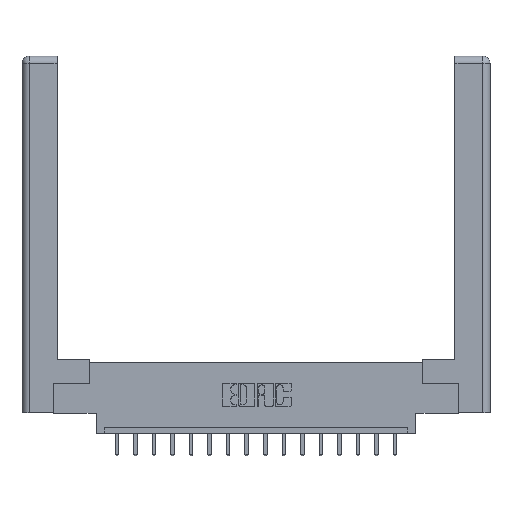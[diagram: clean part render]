
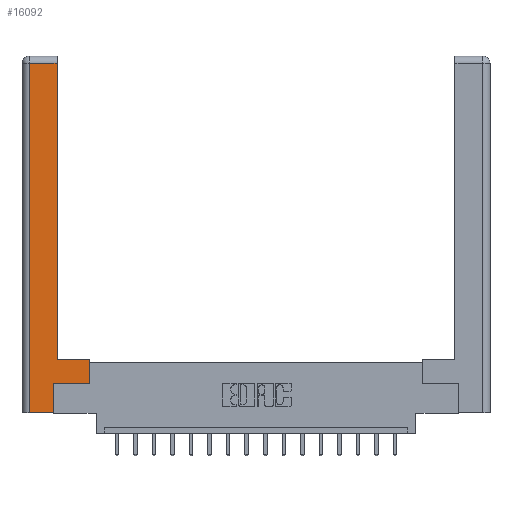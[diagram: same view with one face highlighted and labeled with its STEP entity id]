
A CAD part, top view. The second image highlights one B-rep face of the part: STEP entity #16092.
In plain terms, the highlighted planar face has unit normal (0, 0, 1).
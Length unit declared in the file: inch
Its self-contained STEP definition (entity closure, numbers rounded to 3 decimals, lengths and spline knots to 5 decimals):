
#26 = VECTOR ( 'NONE', #1888, 39.37008 ) ;
#117 = VERTEX_POINT ( 'NONE', #9153 ) ;
#232 = AXIS2_PLACEMENT_3D ( 'NONE', #5688, #18079, #15483 ) ;
#305 = CARTESIAN_POINT ( 'NONE',  ( 0.265, 0.245, 0. ) ) ;
#758 = DIRECTION ( 'NONE',  ( -1., 0., 0. ) ) ;
#790 = ORIENTED_EDGE ( 'NONE', *, *, #12209, .T. ) ;
#1109 = DIRECTION ( 'NONE',  ( -1., 0., 0. ) ) ;
#1177 = CARTESIAN_POINT ( 'NONE',  ( 0.295, 0.45, 0. ) ) ;
#1500 = CARTESIAN_POINT ( 'NONE',  ( 0.565, 0.245, 0. ) ) ;
#1694 = VECTOR ( 'NONE', #3540, 39.37008 ) ;
#1888 = DIRECTION ( 'NONE',  ( 1., 0., 0. ) ) ;
#2169 = LINE ( 'NONE', #305, #2615 ) ;
#2547 = VERTEX_POINT ( 'NONE', #9567 ) ;
#2615 = VECTOR ( 'NONE', #14109, 39.37008 ) ;
#2792 = ORIENTED_EDGE ( 'NONE', *, *, #10986, .T. ) ;
#3011 = CARTESIAN_POINT ( 'NONE',  ( 0.0615, 2.94, 0. ) ) ;
#3387 = CARTESIAN_POINT ( 'NONE',  ( 0.295, 3., 0. ) ) ;
#3540 = DIRECTION ( 'NONE',  ( 0., -1., 0. ) ) ;
#3660 = CARTESIAN_POINT ( 'NONE',  ( 0.0615, 0., 0. ) ) ;
#3812 = DIRECTION ( 'NONE',  ( 0., 1., 0. ) ) ;
#4677 = VECTOR ( 'NONE', #1109, 39.37008 ) ;
#4827 = VECTOR ( 'NONE', #12919, 39.37008 ) ;
#4859 = CARTESIAN_POINT ( 'NONE',  ( 0.295, 2.94, 0. ) ) ;
#4862 = VECTOR ( 'NONE', #758, 39.37008 ) ;
#5351 = CARTESIAN_POINT ( 'NONE',  ( 0.565, 0.245, 0. ) ) ;
#5362 = LINE ( 'NONE', #3387, #5566 ) ;
#5566 = VECTOR ( 'NONE', #7525, 39.37008 ) ;
#5688 = CARTESIAN_POINT ( 'NONE',  ( 0., 0., 0. ) ) ;
#6109 = VERTEX_POINT ( 'NONE', #17851 ) ;
#7306 = LINE ( 'NONE', #13396, #4862 ) ;
#7525 = DIRECTION ( 'NONE',  ( 0., 1., 0. ) ) ;
#7606 = FACE_OUTER_BOUND ( 'NONE', #17423, .T. ) ;
#7648 = ORIENTED_EDGE ( 'NONE', *, *, #13718, .T. ) ;
#8230 = CARTESIAN_POINT ( 'NONE',  ( 0.295, 0.45, 0. ) ) ;
#8294 = EDGE_CURVE ( 'NONE', #6109, #16015, #8418, .T. ) ;
#8418 = LINE ( 'NONE', #1177, #4677 ) ;
#8572 = LINE ( 'NONE', #1500, #4827 ) ;
#8828 = VERTEX_POINT ( 'NONE', #4859 ) ;
#8994 = EDGE_CURVE ( 'NONE', #9132, #6109, #12313, .T. ) ;
#9132 = VERTEX_POINT ( 'NONE', #5351 ) ;
#9153 = CARTESIAN_POINT ( 'NONE',  ( 0.0615, 0., 0. ) ) ;
#9270 = VECTOR ( 'NONE', #3812, 39.37008 ) ;
#9567 = CARTESIAN_POINT ( 'NONE',  ( 0.265, 0., 0. ) ) ;
#9794 = EDGE_CURVE ( 'NONE', #13438, #9132, #8572, .T. ) ;
#10761 = CARTESIAN_POINT ( 'NONE',  ( 0.265, 0.245, 0. ) ) ;
#10986 = EDGE_CURVE ( 'NONE', #16015, #8828, #5362, .T. ) ;
#11499 = VERTEX_POINT ( 'NONE', #3011 ) ;
#11604 = EDGE_CURVE ( 'NONE', #117, #2547, #12328, .T. ) ;
#12047 = ORIENTED_EDGE ( 'NONE', *, *, #14953, .T. ) ;
#12209 = EDGE_CURVE ( 'NONE', #8828, #11499, #7306, .T. ) ;
#12214 = LINE ( 'NONE', #3660, #1694 ) ;
#12313 = LINE ( 'NONE', #16367, #9270 ) ;
#12328 = LINE ( 'NONE', #14703, #26 ) ;
#12919 = DIRECTION ( 'NONE',  ( 1., 0., 0. ) ) ;
#13396 = CARTESIAN_POINT ( 'NONE',  ( 0.0615, 2.94, 0. ) ) ;
#13438 = VERTEX_POINT ( 'NONE', #10761 ) ;
#13718 = EDGE_CURVE ( 'NONE', #2547, #13438, #2169, .T. ) ;
#13885 = PLANE ( 'NONE',  #232 ) ;
#14109 = DIRECTION ( 'NONE',  ( 0., 1., 0. ) ) ;
#14703 = CARTESIAN_POINT ( 'NONE',  ( 0.265, 0., 0. ) ) ;
#14953 = EDGE_CURVE ( 'NONE', #11499, #117, #12214, .T. ) ;
#15483 = DIRECTION ( 'NONE',  ( -1., 0., 0. ) ) ;
#15624 = ORIENTED_EDGE ( 'NONE', *, *, #8294, .T. ) ;
#15806 = ORIENTED_EDGE ( 'NONE', *, *, #11604, .T. ) ;
#15834 = ORIENTED_EDGE ( 'NONE', *, *, #8994, .T. ) ;
#16015 = VERTEX_POINT ( 'NONE', #8230 ) ;
#16092 = ADVANCED_FACE ( 'NONE', ( #7606 ), #13885, .F. ) ;
#16367 = CARTESIAN_POINT ( 'NONE',  ( 0.565, 0.45, 0. ) ) ;
#16828 = ORIENTED_EDGE ( 'NONE', *, *, #9794, .T. ) ;
#17423 = EDGE_LOOP ( 'NONE', ( #2792, #790, #12047, #15806, #7648, #16828, #15834, #15624 ) ) ;
#17851 = CARTESIAN_POINT ( 'NONE',  ( 0.565, 0.45, 0. ) ) ;
#18079 = DIRECTION ( 'NONE',  ( 0., 0., -1. ) ) ;
